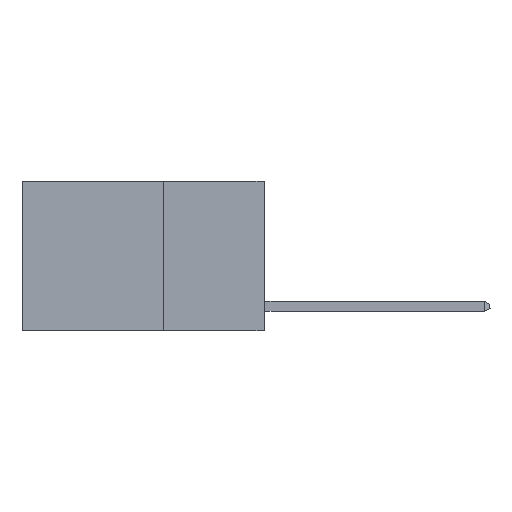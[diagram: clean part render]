
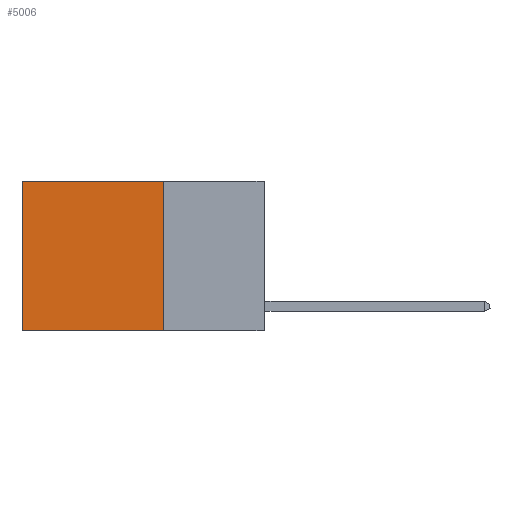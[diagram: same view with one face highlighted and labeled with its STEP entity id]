
A CAD part, left-side view. The second image highlights one B-rep face of the part: STEP entity #5006.
In plain terms, the highlighted planar face has unit normal (-1, 0, 0).
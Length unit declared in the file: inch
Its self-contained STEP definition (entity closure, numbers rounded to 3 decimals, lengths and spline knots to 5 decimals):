
#58 = ORIENTED_EDGE ( 'NONE', *, *, #7200, .F. ) ;
#91 = VECTOR ( 'NONE', #6516, 39.37008 ) ;
#426 = ORIENTED_EDGE ( 'NONE', *, *, #1426, .F. ) ;
#506 = CARTESIAN_POINT ( 'NONE',  ( 0.2625, 0.6, 0. ) ) ;
#591 = DIRECTION ( 'NONE',  ( 0., 0., -1. ) ) ;
#679 = EDGE_CURVE ( 'NONE', #5725, #6206, #5795, .T. ) ;
#971 = CARTESIAN_POINT ( 'NONE',  ( 0.2625, 0.25, 0. ) ) ;
#1373 = CARTESIAN_POINT ( 'NONE',  ( 0.2625, 0.25, 0. ) ) ;
#1415 = CARTESIAN_POINT ( 'NONE',  ( 0.2625, 0.25, 0. ) ) ;
#1426 = EDGE_CURVE ( 'NONE', #4075, #6206, #3219, .T. ) ;
#2240 = LINE ( 'NONE', #1415, #91 ) ;
#2430 = CARTESIAN_POINT ( 'NONE',  ( 0.2625, 0.25, -0.37 ) ) ;
#3098 = VECTOR ( 'NONE', #591, 39.37008 ) ;
#3219 = LINE ( 'NONE', #2430, #8906 ) ;
#3265 = ORIENTED_EDGE ( 'NONE', *, *, #8618, .T. ) ;
#3924 = FACE_OUTER_BOUND ( 'NONE', #7371, .T. ) ;
#4075 = VERTEX_POINT ( 'NONE', #5495 ) ;
#5006 = ADVANCED_FACE ( 'NONE', ( #3924 ), #8064, .F. ) ;
#5475 = CARTESIAN_POINT ( 'NONE',  ( 0.2625, 0.6, -0.37 ) ) ;
#5495 = CARTESIAN_POINT ( 'NONE',  ( 0.2625, 0.25, -0.37 ) ) ;
#5639 = ORIENTED_EDGE ( 'NONE', *, *, #679, .T. ) ;
#5725 = VERTEX_POINT ( 'NONE', #506 ) ;
#5795 = LINE ( 'NONE', #10026, #3098 ) ;
#6052 = DIRECTION ( 'NONE',  ( 0., 1., 0. ) ) ;
#6206 = VERTEX_POINT ( 'NONE', #5475 ) ;
#6497 = CARTESIAN_POINT ( 'NONE',  ( 0.2625, 0.25, 0. ) ) ;
#6516 = DIRECTION ( 'NONE',  ( 0., 0., -1. ) ) ;
#6655 = DIRECTION ( 'NONE',  ( 0., 1., 0. ) ) ;
#6821 = AXIS2_PLACEMENT_3D ( 'NONE', #1373, #9744, #7328 ) ;
#6962 = LINE ( 'NONE', #971, #10603 ) ;
#7200 = EDGE_CURVE ( 'NONE', #7703, #4075, #2240, .T. ) ;
#7328 = DIRECTION ( 'NONE',  ( 0., 0., -1. ) ) ;
#7371 = EDGE_LOOP ( 'NONE', ( #5639, #426, #58, #3265 ) ) ;
#7703 = VERTEX_POINT ( 'NONE', #6497 ) ;
#8064 = PLANE ( 'NONE',  #6821 ) ;
#8618 = EDGE_CURVE ( 'NONE', #7703, #5725, #6962, .T. ) ;
#8906 = VECTOR ( 'NONE', #6655, 39.37008 ) ;
#9744 = DIRECTION ( 'NONE',  ( 1., 0., 0. ) ) ;
#10026 = CARTESIAN_POINT ( 'NONE',  ( 0.2625, 0.6, 0. ) ) ;
#10603 = VECTOR ( 'NONE', #6052, 39.37008 ) ;
